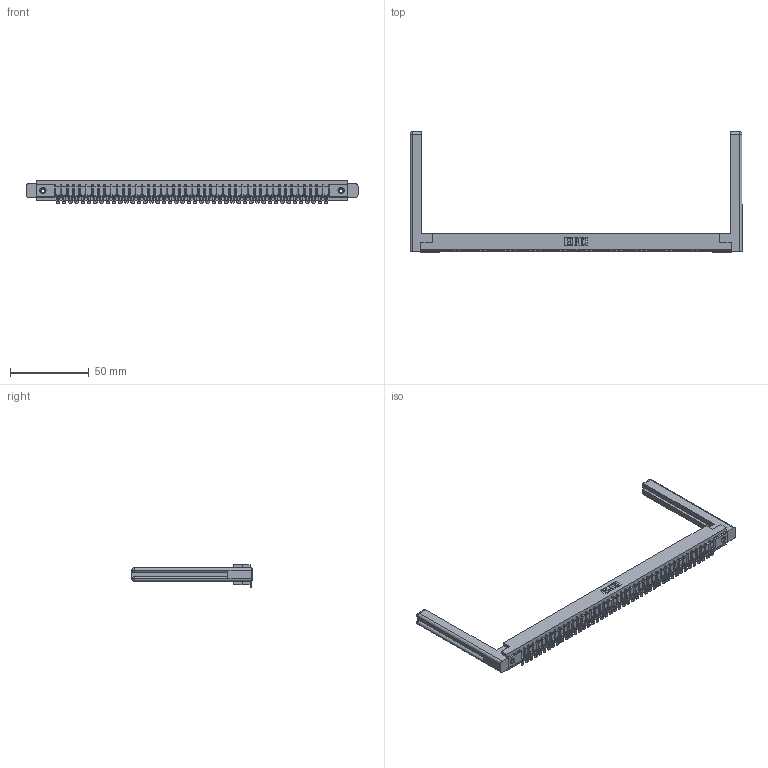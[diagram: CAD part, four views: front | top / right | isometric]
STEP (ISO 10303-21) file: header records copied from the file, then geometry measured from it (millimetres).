
FILE_DESCRIPTION (( 'STEP AP203' ), '1' );
FILE_NAME ('307-044-454-158.STEP', '2020-09-29T23:18:44', ( '' ), ( '' ), 'SwSTEP 2.0', 'SolidWorks 2020', '' );
FILE_SCHEMA (( 'CONFIG_CONTROL_DESIGN' ));
Length unit declared in the file: inch
Products named in the file (5): 307-044-454-158; 307 Part_.156 Dia Mounting Holes; 307-220-058; 345-250-001_345-250-001-102; 307-290-002_554
Assembly tree (49 placements, depth 2):
  307-044-454-158
    307 Part_.156 Dia Mounting Holes
    307-290-002_554  x44
    307-220-058  x2
    345-250-001_345-250-001-102  x2
Bounding box: 210.97 x 76.33 x 14.52 mm (x, y, z)
Volume: 29727.7 mm3; surface area: 33470.6 mm2
Topology: 49 solids, 49 shells, 3869 faces, 11809 edges, 7738 vertices
Faces by surface type: plane 2178, cylinder 1577, sphere 90, torus 12, cone 12
Entity records: 41072 total; most frequent: CARTESIAN_POINT 6937, ORIENTED_EDGE 6866, DIRECTION 6705, EDGE_CURVE 3433, LINE 2621, VECTOR 2621, VERTEX_POINT 2220, AXIS2_PLACEMENT_3D 2042
